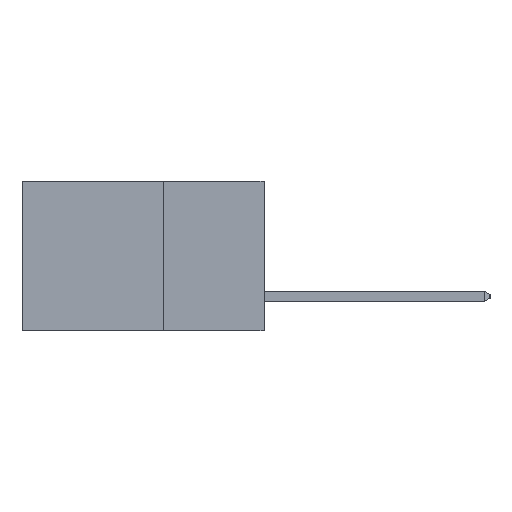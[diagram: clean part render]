
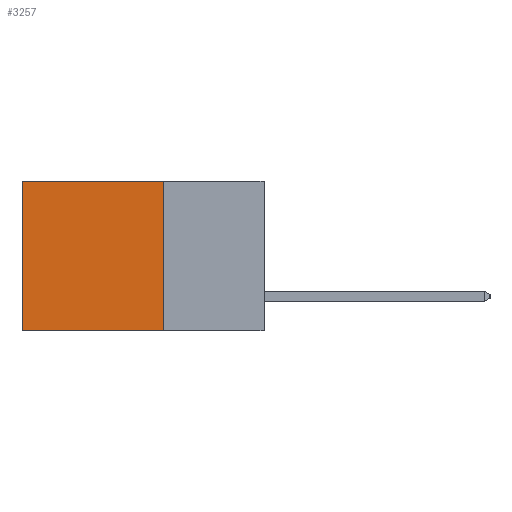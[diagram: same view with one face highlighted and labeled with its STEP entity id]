
A CAD part, left-side view. The second image highlights one B-rep face of the part: STEP entity #3257.
In plain terms, the highlighted planar face has unit normal (-1, 0, 0).
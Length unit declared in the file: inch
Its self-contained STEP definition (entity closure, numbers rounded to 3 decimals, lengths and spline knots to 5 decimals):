
#119 = DIRECTION ( 'NONE',  ( 0., 0., -1. ) ) ;
#282 = VERTEX_POINT ( 'NONE', #4550 ) ;
#376 = CARTESIAN_POINT ( 'NONE',  ( 0.2615, 0.25, -0.37 ) ) ;
#632 = CARTESIAN_POINT ( 'NONE',  ( 0.2615, 0.25, 0. ) ) ;
#1901 = ORIENTED_EDGE ( 'NONE', *, *, #2613, .F. ) ;
#2046 = LINE ( 'NONE', #6636, #5575 ) ;
#2589 = VERTEX_POINT ( 'NONE', #4144 ) ;
#2613 = EDGE_CURVE ( 'NONE', #282, #2589, #2046, .T. ) ;
#2674 = LINE ( 'NONE', #3830, #7937 ) ;
#2732 = DIRECTION ( 'NONE',  ( 0., 1., 0. ) ) ;
#3228 = LINE ( 'NONE', #7045, #8463 ) ;
#3257 = ADVANCED_FACE ( 'NONE', ( #3997 ), #5883, .F. ) ;
#3277 = ORIENTED_EDGE ( 'NONE', *, *, #3848, .T. ) ;
#3410 = ORIENTED_EDGE ( 'NONE', *, *, #8021, .F. ) ;
#3830 = CARTESIAN_POINT ( 'NONE',  ( 0.2615, 0.6, -0.37 ) ) ;
#3848 = EDGE_CURVE ( 'NONE', #4557, #2589, #2674, .T. ) ;
#3959 = DIRECTION ( 'NONE',  ( 0., 0., -1. ) ) ;
#3997 = FACE_OUTER_BOUND ( 'NONE', #4729, .T. ) ;
#4144 = CARTESIAN_POINT ( 'NONE',  ( 0.2615, 0.6, -0.37 ) ) ;
#4524 = VECTOR ( 'NONE', #6771, 39.37008 ) ;
#4550 = CARTESIAN_POINT ( 'NONE',  ( 0.2615, 0.25, -0.37 ) ) ;
#4557 = VERTEX_POINT ( 'NONE', #6826 ) ;
#4576 = ORIENTED_EDGE ( 'NONE', *, *, #6110, .T. ) ;
#4729 = EDGE_LOOP ( 'NONE', ( #3277, #1901, #3410, #4576 ) ) ;
#4736 = LINE ( 'NONE', #5517, #4524 ) ;
#5366 = DIRECTION ( 'NONE',  ( 0., 0., -1. ) ) ;
#5400 = DIRECTION ( 'NONE',  ( 1., 0., 0. ) ) ;
#5517 = CARTESIAN_POINT ( 'NONE',  ( 0.2615, 0.25, 0. ) ) ;
#5575 = VECTOR ( 'NONE', #2732, 39.37008 ) ;
#5883 = PLANE ( 'NONE',  #7298 ) ;
#6110 = EDGE_CURVE ( 'NONE', #7908, #4557, #4736, .T. ) ;
#6636 = CARTESIAN_POINT ( 'NONE',  ( 0.2615, 0.25, -0.37 ) ) ;
#6771 = DIRECTION ( 'NONE',  ( 0., 1., 0. ) ) ;
#6826 = CARTESIAN_POINT ( 'NONE',  ( 0.2615, 0.6, 0. ) ) ;
#7045 = CARTESIAN_POINT ( 'NONE',  ( 0.2615, 0.25, -0.37 ) ) ;
#7298 = AXIS2_PLACEMENT_3D ( 'NONE', #376, #5400, #5366 ) ;
#7908 = VERTEX_POINT ( 'NONE', #632 ) ;
#7937 = VECTOR ( 'NONE', #3959, 39.37008 ) ;
#8021 = EDGE_CURVE ( 'NONE', #7908, #282, #3228, .T. ) ;
#8463 = VECTOR ( 'NONE', #119, 39.37008 ) ;
